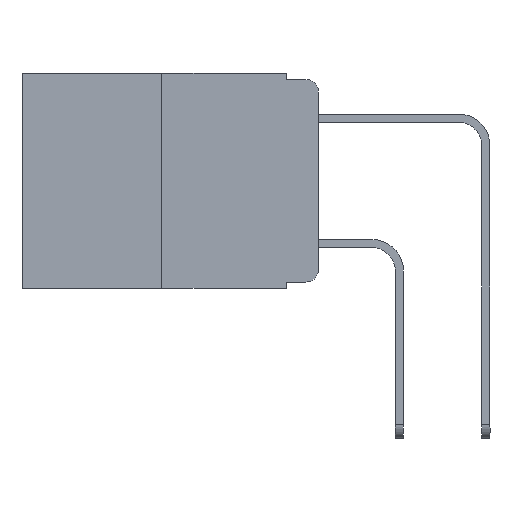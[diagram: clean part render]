
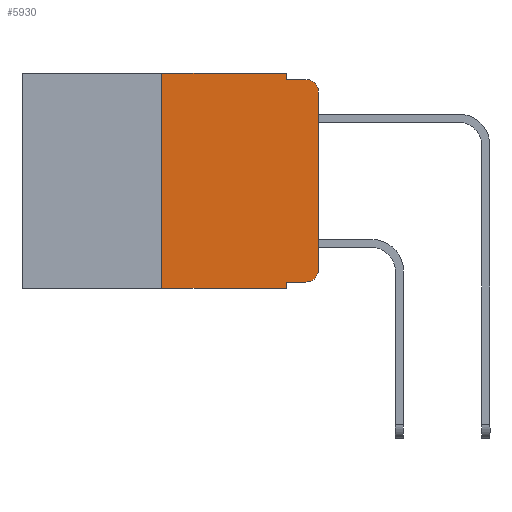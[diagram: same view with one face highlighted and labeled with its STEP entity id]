
A CAD part, left-side view. The second image highlights one B-rep face of the part: STEP entity #5930.
In plain terms, the highlighted planar face has unit normal (-1, 0, 0).
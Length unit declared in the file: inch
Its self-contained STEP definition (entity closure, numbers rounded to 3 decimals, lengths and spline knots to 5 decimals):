
#33 = CARTESIAN_POINT ( 'NONE',  ( 0., 0., -0.313 ) ) ;
#266 = VECTOR ( 'NONE', #3382, 39.37008 ) ;
#329 = VERTEX_POINT ( 'NONE', #6595 ) ;
#442 = ORIENTED_EDGE ( 'NONE', *, *, #4235, .T. ) ;
#447 = DIRECTION ( 'NONE',  ( 0., 0., -1. ) ) ;
#465 = VERTEX_POINT ( 'NONE', #8070 ) ;
#557 = DIRECTION ( 'NONE',  ( 0., -1., 0. ) ) ;
#860 = DIRECTION ( 'NONE',  ( 0., -1., 0. ) ) ;
#1179 = CARTESIAN_POINT ( 'NONE',  ( 0., 0., -0.03 ) ) ;
#1354 = VERTEX_POINT ( 'NONE', #11648 ) ;
#1466 = CARTESIAN_POINT ( 'NONE',  ( 0., 0.25, 0. ) ) ;
#1594 = CARTESIAN_POINT ( 'NONE',  ( 0., 0.051, 0. ) ) ;
#1602 = VERTEX_POINT ( 'NONE', #6722 ) ;
#1626 = CARTESIAN_POINT ( 'NONE',  ( 0., 0.473, -0.343 ) ) ;
#1678 = EDGE_LOOP ( 'NONE', ( #5451, #442, #9276, #8596, #1794, #2656, #3838, #2499, #9426, #7487 ) ) ;
#1794 = ORIENTED_EDGE ( 'NONE', *, *, #10559, .F. ) ;
#1828 = CARTESIAN_POINT ( 'NONE',  ( 0., 0.25, 0. ) ) ;
#2012 = VERTEX_POINT ( 'NONE', #1828 ) ;
#2330 = CARTESIAN_POINT ( 'NONE',  ( 0., 0.02, -0.03 ) ) ;
#2334 = AXIS2_PLACEMENT_3D ( 'NONE', #12013, #4299, #8112 ) ;
#2499 = ORIENTED_EDGE ( 'NONE', *, *, #7174, .F. ) ;
#2534 = LINE ( 'NONE', #1626, #7215 ) ;
#2656 = ORIENTED_EDGE ( 'NONE', *, *, #9937, .F. ) ;
#2834 = VERTEX_POINT ( 'NONE', #9991 ) ;
#3293 = EDGE_CURVE ( 'NONE', #6482, #12104, #11877, .T. ) ;
#3324 = CARTESIAN_POINT ( 'NONE',  ( 0., 0.051, 0. ) ) ;
#3382 = DIRECTION ( 'NONE',  ( 0., -1., 0. ) ) ;
#3838 = ORIENTED_EDGE ( 'NONE', *, *, #5187, .T. ) ;
#4235 = EDGE_CURVE ( 'NONE', #12104, #1602, #10729, .T. ) ;
#4252 = DIRECTION ( 'NONE',  ( 0., 0., -1. ) ) ;
#4281 = DIRECTION ( 'NONE',  ( 0., 0., 1. ) ) ;
#4299 = DIRECTION ( 'NONE',  ( -1., 0., 0. ) ) ;
#4512 = LINE ( 'NONE', #5515, #5164 ) ;
#4737 = VECTOR ( 'NONE', #7109, 39.37008 ) ;
#4994 = VERTEX_POINT ( 'NONE', #7898 ) ;
#5062 = PLANE ( 'NONE',  #5490 ) ;
#5164 = VECTOR ( 'NONE', #860, 39.37008 ) ;
#5166 = CARTESIAN_POINT ( 'NONE',  ( 0., 0.051, -0.01 ) ) ;
#5187 = EDGE_CURVE ( 'NONE', #2834, #1354, #2534, .T. ) ;
#5365 = LINE ( 'NONE', #11947, #266 ) ;
#5370 = CARTESIAN_POINT ( 'NONE',  ( 0., 0.473, 0. ) ) ;
#5399 = DIRECTION ( 'NONE',  ( 0., -1., 0. ) ) ;
#5451 = ORIENTED_EDGE ( 'NONE', *, *, #3293, .T. ) ;
#5490 = AXIS2_PLACEMENT_3D ( 'NONE', #5370, #9000, #8056 ) ;
#5515 = CARTESIAN_POINT ( 'NONE',  ( 0., 0.473, 0. ) ) ;
#5930 = ADVANCED_FACE ( 'NONE', ( #9801 ), #5062, .F. ) ;
#6010 = VERTEX_POINT ( 'NONE', #3324 ) ;
#6033 = DIRECTION ( 'NONE',  ( 0., 0., -1. ) ) ;
#6482 = VERTEX_POINT ( 'NONE', #33 ) ;
#6595 = CARTESIAN_POINT ( 'NONE',  ( 0., 0.02, -0.333 ) ) ;
#6722 = CARTESIAN_POINT ( 'NONE',  ( 0., 0.02, -0.01 ) ) ;
#6987 = EDGE_CURVE ( 'NONE', #465, #329, #5365, .T. ) ;
#7109 = DIRECTION ( 'NONE',  ( 0., 0., 1. ) ) ;
#7174 = EDGE_CURVE ( 'NONE', #465, #1354, #10741, .T. ) ;
#7199 = DIRECTION ( 'NONE',  ( -1., 0., 0. ) ) ;
#7215 = VECTOR ( 'NONE', #5399, 39.37008 ) ;
#7228 = LINE ( 'NONE', #5166, #9563 ) ;
#7487 = ORIENTED_EDGE ( 'NONE', *, *, #8255, .T. ) ;
#7898 = CARTESIAN_POINT ( 'NONE',  ( 0., 0.051, -0.01 ) ) ;
#8056 = DIRECTION ( 'NONE',  ( 0., 0., -1. ) ) ;
#8070 = CARTESIAN_POINT ( 'NONE',  ( 0., 0.051, -0.333 ) ) ;
#8102 = VECTOR ( 'NONE', #447, 39.37008 ) ;
#8112 = DIRECTION ( 'NONE',  ( 0., 0., -1. ) ) ;
#8240 = EDGE_CURVE ( 'NONE', #6010, #4994, #12132, .T. ) ;
#8255 = EDGE_CURVE ( 'NONE', #329, #6482, #11731, .T. ) ;
#8596 = ORIENTED_EDGE ( 'NONE', *, *, #8240, .F. ) ;
#8672 = VECTOR ( 'NONE', #6033, 39.37008 ) ;
#9000 = DIRECTION ( 'NONE',  ( 1., 0., 0. ) ) ;
#9112 = LINE ( 'NONE', #1466, #4737 ) ;
#9149 = AXIS2_PLACEMENT_3D ( 'NONE', #2330, #7199, #4252 ) ;
#9276 = ORIENTED_EDGE ( 'NONE', *, *, #11217, .F. ) ;
#9426 = ORIENTED_EDGE ( 'NONE', *, *, #6987, .T. ) ;
#9563 = VECTOR ( 'NONE', #557, 39.37008 ) ;
#9801 = FACE_OUTER_BOUND ( 'NONE', #1678, .T. ) ;
#9937 = EDGE_CURVE ( 'NONE', #2834, #2012, #9112, .T. ) ;
#9991 = CARTESIAN_POINT ( 'NONE',  ( 0., 0.25, -0.343 ) ) ;
#10220 = CARTESIAN_POINT ( 'NONE',  ( 0., 0., 0. ) ) ;
#10559 = EDGE_CURVE ( 'NONE', #2012, #6010, #4512, .T. ) ;
#10729 = CIRCLE ( 'NONE', #9149, 0.02 ) ;
#10741 = LINE ( 'NONE', #11512, #8672 ) ;
#11217 = EDGE_CURVE ( 'NONE', #4994, #1602, #7228, .T. ) ;
#11512 = CARTESIAN_POINT ( 'NONE',  ( 0., 0.051, 0. ) ) ;
#11648 = CARTESIAN_POINT ( 'NONE',  ( 0., 0.051, -0.343 ) ) ;
#11731 = CIRCLE ( 'NONE', #2334, 0.02 ) ;
#11877 = LINE ( 'NONE', #10220, #12236 ) ;
#11947 = CARTESIAN_POINT ( 'NONE',  ( 0., 0.051, -0.333 ) ) ;
#12013 = CARTESIAN_POINT ( 'NONE',  ( 0., 0.02, -0.313 ) ) ;
#12104 = VERTEX_POINT ( 'NONE', #1179 ) ;
#12132 = LINE ( 'NONE', #1594, #8102 ) ;
#12236 = VECTOR ( 'NONE', #4281, 39.37008 ) ;
